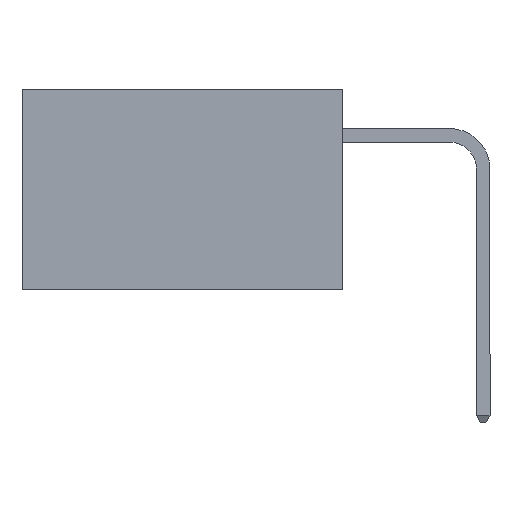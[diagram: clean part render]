
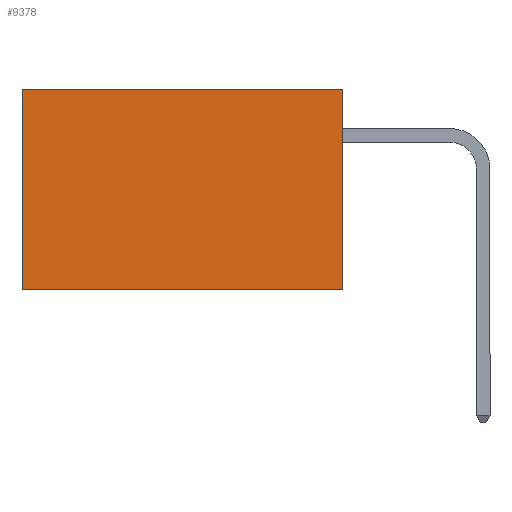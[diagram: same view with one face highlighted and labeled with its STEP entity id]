
A CAD part, left-side view. The second image highlights one B-rep face of the part: STEP entity #9378.
In plain terms, the highlighted planar face has unit normal (-1, 0, 0).
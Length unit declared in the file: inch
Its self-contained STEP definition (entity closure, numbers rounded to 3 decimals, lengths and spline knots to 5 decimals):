
#51 = ORIENTED_EDGE ( 'NONE', *, *, #9156, .F. ) ;
#906 = CARTESIAN_POINT ( 'NONE',  ( 0.277, 0., 0. ) ) ;
#1989 = CARTESIAN_POINT ( 'NONE',  ( 0.277, 0., -0.37 ) ) ;
#1998 = CARTESIAN_POINT ( 'NONE',  ( 0.277, 0.59, -0.37 ) ) ;
#2053 = VECTOR ( 'NONE', #8254, 39.37008 ) ;
#2498 = VECTOR ( 'NONE', #7504, 39.37008 ) ;
#2779 = LINE ( 'NONE', #1998, #7417 ) ;
#2898 = DIRECTION ( 'NONE',  ( 0., 0., -1. ) ) ;
#3311 = DIRECTION ( 'NONE',  ( 0., 0., -1. ) ) ;
#4121 = CARTESIAN_POINT ( 'NONE',  ( 0.277, 0.59, -0.37 ) ) ;
#4263 = AXIS2_PLACEMENT_3D ( 'NONE', #6981, #8821, #3311 ) ;
#4419 = VERTEX_POINT ( 'NONE', #4121 ) ;
#4665 = VECTOR ( 'NONE', #7451, 39.37008 ) ;
#4691 = CARTESIAN_POINT ( 'NONE',  ( 0.277, 0., 0. ) ) ;
#4878 = EDGE_CURVE ( 'NONE', #8529, #9738, #7088, .T. ) ;
#5270 = LINE ( 'NONE', #8441, #2498 ) ;
#5421 = VERTEX_POINT ( 'NONE', #6363 ) ;
#6363 = CARTESIAN_POINT ( 'NONE',  ( 0.277, 0.59, 0. ) ) ;
#6667 = CARTESIAN_POINT ( 'NONE',  ( 0.277, 0., -0.37 ) ) ;
#6949 = LINE ( 'NONE', #906, #2053 ) ;
#6968 = EDGE_LOOP ( 'NONE', ( #8725, #51, #9252, #10796 ) ) ;
#6981 = CARTESIAN_POINT ( 'NONE',  ( 0.277, 0., -0.37 ) ) ;
#7088 = LINE ( 'NONE', #6667, #4665 ) ;
#7417 = VECTOR ( 'NONE', #2898, 39.37008 ) ;
#7451 = DIRECTION ( 'NONE',  ( 0., 0., -1. ) ) ;
#7504 = DIRECTION ( 'NONE',  ( 0., 1., 0. ) ) ;
#7919 = PLANE ( 'NONE',  #4263 ) ;
#8254 = DIRECTION ( 'NONE',  ( 0., 1., 0. ) ) ;
#8441 = CARTESIAN_POINT ( 'NONE',  ( 0.277, 0., -0.37 ) ) ;
#8529 = VERTEX_POINT ( 'NONE', #4691 ) ;
#8725 = ORIENTED_EDGE ( 'NONE', *, *, #9150, .T. ) ;
#8821 = DIRECTION ( 'NONE',  ( 1., 0., 0. ) ) ;
#9150 = EDGE_CURVE ( 'NONE', #5421, #4419, #2779, .T. ) ;
#9156 = EDGE_CURVE ( 'NONE', #9738, #4419, #5270, .T. ) ;
#9252 = ORIENTED_EDGE ( 'NONE', *, *, #4878, .F. ) ;
#9378 = ADVANCED_FACE ( 'NONE', ( #11853 ), #7919, .F. ) ;
#9738 = VERTEX_POINT ( 'NONE', #1989 ) ;
#10281 = EDGE_CURVE ( 'NONE', #8529, #5421, #6949, .T. ) ;
#10796 = ORIENTED_EDGE ( 'NONE', *, *, #10281, .T. ) ;
#11853 = FACE_OUTER_BOUND ( 'NONE', #6968, .T. ) ;
